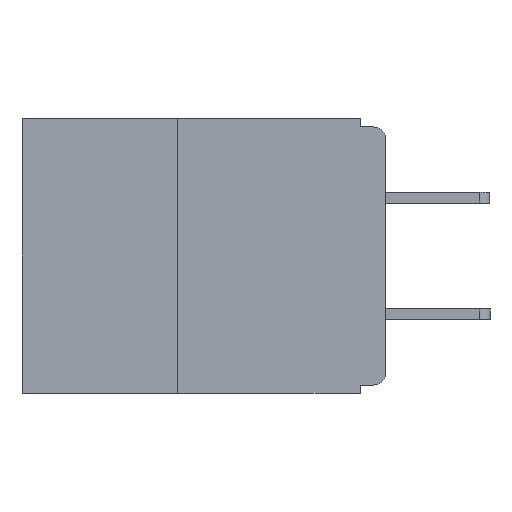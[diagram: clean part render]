
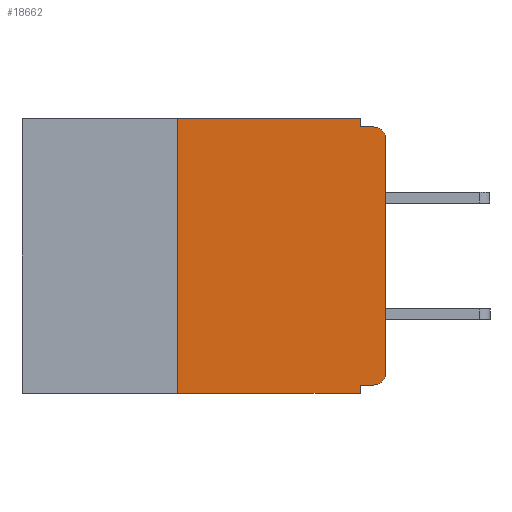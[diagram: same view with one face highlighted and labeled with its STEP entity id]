
A CAD part, left-side view. The second image highlights one B-rep face of the part: STEP entity #18662.
In plain terms, the highlighted planar face has unit normal (-1, 0, 0).
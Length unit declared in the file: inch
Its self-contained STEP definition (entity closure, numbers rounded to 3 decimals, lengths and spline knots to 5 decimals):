
#1181 = VERTEX_POINT ( 'NONE', #6055 ) ;
#1472 = DIRECTION ( 'NONE',  ( 0., 0., 1. ) ) ;
#1553 = ORIENTED_EDGE ( 'NONE', *, *, #11382, .T. ) ;
#1569 = CARTESIAN_POINT ( 'NONE',  ( 0., 0., 0. ) ) ;
#2000 = DIRECTION ( 'NONE',  ( 0., -1., 0. ) ) ;
#2743 = LINE ( 'NONE', #26285, #25356 ) ;
#3199 = EDGE_CURVE ( 'NONE', #4177, #1181, #2743, .T. ) ;
#3321 = ORIENTED_EDGE ( 'NONE', *, *, #5009, .T. ) ;
#4046 = LINE ( 'NONE', #1569, #20256 ) ;
#4177 = VERTEX_POINT ( 'NONE', #13117 ) ;
#4181 = LINE ( 'NONE', #6730, #19689 ) ;
#4272 = CARTESIAN_POINT ( 'NONE',  ( 0., 0.437, 0. ) ) ;
#5009 = EDGE_CURVE ( 'NONE', #6239, #8315, #4046, .T. ) ;
#5331 = LINE ( 'NONE', #20610, #27699 ) ;
#5424 = ORIENTED_EDGE ( 'NONE', *, *, #5449, .F. ) ;
#5449 = EDGE_CURVE ( 'NONE', #22415, #6213, #6365, .T. ) ;
#5587 = EDGE_CURVE ( 'NONE', #12505, #12962, #4181, .T. ) ;
#5760 = DIRECTION ( 'NONE',  ( 0., 0., -1. ) ) ;
#5848 = DIRECTION ( 'NONE',  ( 0., 0., 1. ) ) ;
#6055 = CARTESIAN_POINT ( 'NONE',  ( 0., 0.015, -0.01 ) ) ;
#6213 = VERTEX_POINT ( 'NONE', #18714 ) ;
#6239 = VERTEX_POINT ( 'NONE', #18290 ) ;
#6365 = LINE ( 'NONE', #14003, #11640 ) ;
#6603 = CARTESIAN_POINT ( 'NONE',  ( 0., 0.015, -0.025 ) ) ;
#6676 = CARTESIAN_POINT ( 'NONE',  ( 0., 0.015, -0.32 ) ) ;
#6730 = CARTESIAN_POINT ( 'NONE',  ( 0., 0.25, -0.33 ) ) ;
#6827 = CARTESIAN_POINT ( 'NONE',  ( 0., 0.031, -0.32 ) ) ;
#7248 = VECTOR ( 'NONE', #10415, 39.37008 ) ;
#8110 = ORIENTED_EDGE ( 'NONE', *, *, #5587, .F. ) ;
#8315 = VERTEX_POINT ( 'NONE', #20860 ) ;
#8344 = ORIENTED_EDGE ( 'NONE', *, *, #15620, .T. ) ;
#8569 = CARTESIAN_POINT ( 'NONE',  ( 0., 0.25, -0.33 ) ) ;
#8691 = LINE ( 'NONE', #12555, #7248 ) ;
#8906 = DIRECTION ( 'NONE',  ( 0., 0., -1. ) ) ;
#9067 = EDGE_CURVE ( 'NONE', #23513, #22415, #8691, .T. ) ;
#9505 = AXIS2_PLACEMENT_3D ( 'NONE', #6603, #21898, #8906 ) ;
#10034 = ORIENTED_EDGE ( 'NONE', *, *, #9067, .F. ) ;
#10361 = PLANE ( 'NONE',  #12454 ) ;
#10415 = DIRECTION ( 'NONE',  ( 0., 1., 0. ) ) ;
#10418 = ORIENTED_EDGE ( 'NONE', *, *, #10494, .F. ) ;
#10494 = EDGE_CURVE ( 'NONE', #14233, #4177, #27399, .T. ) ;
#11382 = EDGE_CURVE ( 'NONE', #8315, #1181, #21794, .T. ) ;
#11640 = VECTOR ( 'NONE', #14338, 39.37008 ) ;
#11896 = DIRECTION ( 'NONE',  ( -1., 0., 0. ) ) ;
#11968 = ORIENTED_EDGE ( 'NONE', *, *, #21954, .T. ) ;
#12294 = LINE ( 'NONE', #4272, #23033 ) ;
#12454 = AXIS2_PLACEMENT_3D ( 'NONE', #18962, #25392, #12595 ) ;
#12505 = VERTEX_POINT ( 'NONE', #8569 ) ;
#12555 = CARTESIAN_POINT ( 'NONE',  ( 0., 0., -0.32 ) ) ;
#12595 = DIRECTION ( 'NONE',  ( 0., 0., -1. ) ) ;
#12962 = VERTEX_POINT ( 'NONE', #14496 ) ;
#13117 = CARTESIAN_POINT ( 'NONE',  ( 0., 0.031, -0.01 ) ) ;
#13120 = CARTESIAN_POINT ( 'NONE',  ( 0., 0.031, 0. ) ) ;
#13591 = EDGE_CURVE ( 'NONE', #12962, #14233, #12294, .T. ) ;
#13953 = FACE_OUTER_BOUND ( 'NONE', #25457, .T. ) ;
#14003 = CARTESIAN_POINT ( 'NONE',  ( 0., 0.031, -0.33 ) ) ;
#14233 = VERTEX_POINT ( 'NONE', #13120 ) ;
#14338 = DIRECTION ( 'NONE',  ( 0., 0., -1. ) ) ;
#14496 = CARTESIAN_POINT ( 'NONE',  ( 0., 0.25, 0. ) ) ;
#15620 = EDGE_CURVE ( 'NONE', #23513, #6239, #17527, .T. ) ;
#17527 = CIRCLE ( 'NONE', #19379, 0.015 ) ;
#18290 = CARTESIAN_POINT ( 'NONE',  ( 0., 0., -0.305 ) ) ;
#18662 = ADVANCED_FACE ( 'NONE', ( #13953 ), #10361, .F. ) ;
#18714 = CARTESIAN_POINT ( 'NONE',  ( 0., 0.031, -0.33 ) ) ;
#18962 = CARTESIAN_POINT ( 'NONE',  ( 0., 0.437, 0. ) ) ;
#19379 = AXIS2_PLACEMENT_3D ( 'NONE', #24745, #11896, #26822 ) ;
#19689 = VECTOR ( 'NONE', #5848, 39.37008 ) ;
#20256 = VECTOR ( 'NONE', #1472, 39.37008 ) ;
#20511 = DIRECTION ( 'NONE',  ( 0., -1., 0. ) ) ;
#20610 = CARTESIAN_POINT ( 'NONE',  ( 0., 0.437, -0.33 ) ) ;
#20860 = CARTESIAN_POINT ( 'NONE',  ( 0., 0., -0.025 ) ) ;
#21794 = CIRCLE ( 'NONE', #9505, 0.015 ) ;
#21847 = VECTOR ( 'NONE', #5760, 39.37008 ) ;
#21898 = DIRECTION ( 'NONE',  ( -1., 0., 0. ) ) ;
#21954 = EDGE_CURVE ( 'NONE', #12505, #6213, #5331, .T. ) ;
#22415 = VERTEX_POINT ( 'NONE', #6827 ) ;
#23033 = VECTOR ( 'NONE', #2000, 39.37008 ) ;
#23513 = VERTEX_POINT ( 'NONE', #6676 ) ;
#24745 = CARTESIAN_POINT ( 'NONE',  ( 0., 0.015, -0.305 ) ) ;
#25267 = CARTESIAN_POINT ( 'NONE',  ( 0., 0.031, 0. ) ) ;
#25356 = VECTOR ( 'NONE', #26108, 39.37008 ) ;
#25392 = DIRECTION ( 'NONE',  ( 1., 0., 0. ) ) ;
#25457 = EDGE_LOOP ( 'NONE', ( #3321, #1553, #28156, #10418, #26950, #8110, #11968, #5424, #10034, #8344 ) ) ;
#26108 = DIRECTION ( 'NONE',  ( 0., -1., 0. ) ) ;
#26285 = CARTESIAN_POINT ( 'NONE',  ( 0., 0., -0.01 ) ) ;
#26822 = DIRECTION ( 'NONE',  ( 0., 0., -1. ) ) ;
#26950 = ORIENTED_EDGE ( 'NONE', *, *, #13591, .F. ) ;
#27399 = LINE ( 'NONE', #25267, #21847 ) ;
#27699 = VECTOR ( 'NONE', #20511, 39.37008 ) ;
#28156 = ORIENTED_EDGE ( 'NONE', *, *, #3199, .F. ) ;
